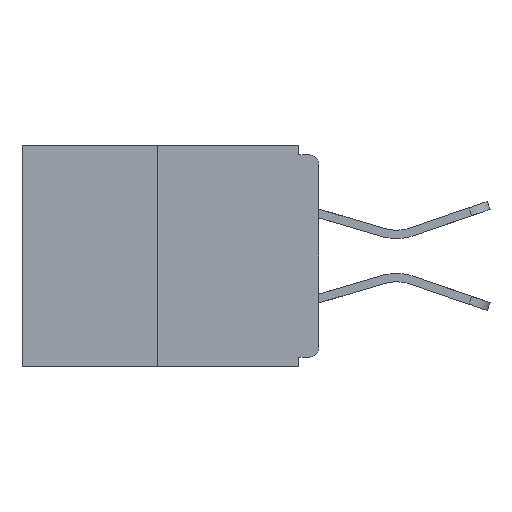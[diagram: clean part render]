
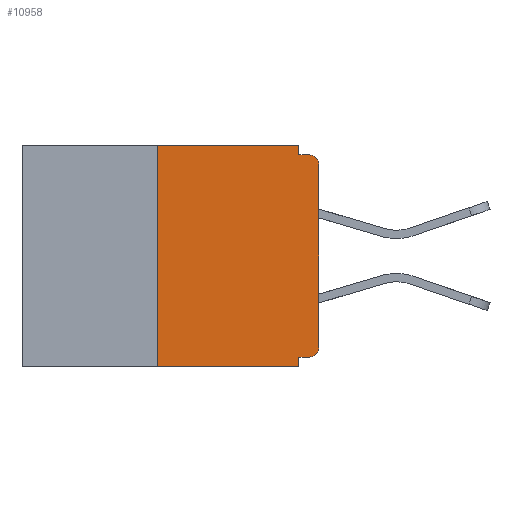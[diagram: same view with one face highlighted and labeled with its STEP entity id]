
A CAD part, left-side view. The second image highlights one B-rep face of the part: STEP entity #10958.
In plain terms, the highlighted planar face has unit normal (-1, 0, 0).
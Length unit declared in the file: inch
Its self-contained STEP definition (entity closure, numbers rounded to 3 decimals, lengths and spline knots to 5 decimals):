
#30 = VERTEX_POINT ( 'NONE', #23460 ) ;
#964 = AXIS2_PLACEMENT_3D ( 'NONE', #13225, #19103, #20833 ) ;
#1089 = VERTEX_POINT ( 'NONE', #25405 ) ;
#2059 = VECTOR ( 'NONE', #21796, 39.37008 ) ;
#2412 = VECTOR ( 'NONE', #14041, 39.37008 ) ;
#2723 = ORIENTED_EDGE ( 'NONE', *, *, #23331, .F. ) ;
#2793 = EDGE_CURVE ( 'NONE', #17201, #6545, #22233, .T. ) ;
#3294 = FACE_OUTER_BOUND ( 'NONE', #9768, .T. ) ;
#3352 = EDGE_CURVE ( 'NONE', #30, #1089, #16151, .T. ) ;
#3661 = CARTESIAN_POINT ( 'NONE',  ( 0., 0.015, -0.328 ) ) ;
#4598 = ORIENTED_EDGE ( 'NONE', *, *, #22551, .F. ) ;
#5006 = VECTOR ( 'NONE', #12530, 39.37008 ) ;
#5181 = DIRECTION ( 'NONE',  ( 0., 1., 0. ) ) ;
#5826 = VECTOR ( 'NONE', #22575, 39.37008 ) ;
#6290 = LINE ( 'NONE', #10565, #2412 ) ;
#6545 = VERTEX_POINT ( 'NONE', #8564 ) ;
#6872 = EDGE_CURVE ( 'NONE', #12479, #18015, #6290, .T. ) ;
#7161 = EDGE_CURVE ( 'NONE', #14339, #30, #17346, .T. ) ;
#7478 = DIRECTION ( 'NONE',  ( 0., 0., -1. ) ) ;
#7545 = PLANE ( 'NONE',  #19122 ) ;
#7570 = VERTEX_POINT ( 'NONE', #12518 ) ;
#7670 = CARTESIAN_POINT ( 'NONE',  ( 0., 0.46, 0. ) ) ;
#7829 = LINE ( 'NONE', #21703, #19369 ) ;
#7931 = DIRECTION ( 'NONE',  ( 0., 0., -1. ) ) ;
#8564 = CARTESIAN_POINT ( 'NONE',  ( 0., 0.015, -0.015 ) ) ;
#9344 = CARTESIAN_POINT ( 'NONE',  ( 0., 0.25, -0.343 ) ) ;
#9361 = ORIENTED_EDGE ( 'NONE', *, *, #24961, .T. ) ;
#9396 = ORIENTED_EDGE ( 'NONE', *, *, #2793, .T. ) ;
#9607 = CIRCLE ( 'NONE', #21958, 0.015 ) ;
#9642 = ORIENTED_EDGE ( 'NONE', *, *, #11290, .F. ) ;
#9716 = DIRECTION ( 'NONE',  ( 0., 0., 1. ) ) ;
#9768 = EDGE_LOOP ( 'NONE', ( #4598, #9642, #13772, #24468, #18959, #16604, #9361, #9396, #2723, #16376 ) ) ;
#9781 = VECTOR ( 'NONE', #24230, 39.37008 ) ;
#10565 = CARTESIAN_POINT ( 'NONE',  ( 0., 0.031, 0. ) ) ;
#10653 = CARTESIAN_POINT ( 'NONE',  ( 0., 0., -0.015 ) ) ;
#10958 = ADVANCED_FACE ( 'NONE', ( #3294 ), #7545, .F. ) ;
#11192 = DIRECTION ( 'NONE',  ( 0., 0., -1. ) ) ;
#11290 = EDGE_CURVE ( 'NONE', #21255, #24212, #7829, .T. ) ;
#11417 = LINE ( 'NONE', #21669, #2059 ) ;
#11774 = CARTESIAN_POINT ( 'NONE',  ( 0., 0., -0.03 ) ) ;
#12479 = VERTEX_POINT ( 'NONE', #24342 ) ;
#12518 = CARTESIAN_POINT ( 'NONE',  ( 0., 0., -0.313 ) ) ;
#12530 = DIRECTION ( 'NONE',  ( 0., -1., 0. ) ) ;
#13225 = CARTESIAN_POINT ( 'NONE',  ( 0., 0.015, -0.03 ) ) ;
#13479 = CARTESIAN_POINT ( 'NONE',  ( 0., 0.015, -0.313 ) ) ;
#13772 = ORIENTED_EDGE ( 'NONE', *, *, #23390, .T. ) ;
#13831 = DIRECTION ( 'NONE',  ( 1., 0., 0. ) ) ;
#13935 = VECTOR ( 'NONE', #5181, 39.37008 ) ;
#14041 = DIRECTION ( 'NONE',  ( 0., 0., -1. ) ) ;
#14100 = CARTESIAN_POINT ( 'NONE',  ( 0., 0., 0. ) ) ;
#14339 = VERTEX_POINT ( 'NONE', #3661 ) ;
#14469 = CARTESIAN_POINT ( 'NONE',  ( 0., 0.46, 0. ) ) ;
#15831 = CARTESIAN_POINT ( 'NONE',  ( 0., 0.031, -0.015 ) ) ;
#16151 = LINE ( 'NONE', #24278, #16752 ) ;
#16205 = EDGE_CURVE ( 'NONE', #14339, #7570, #9607, .T. ) ;
#16376 = ORIENTED_EDGE ( 'NONE', *, *, #6872, .F. ) ;
#16604 = ORIENTED_EDGE ( 'NONE', *, *, #16205, .T. ) ;
#16752 = VECTOR ( 'NONE', #7478, 39.37008 ) ;
#17201 = VERTEX_POINT ( 'NONE', #11774 ) ;
#17346 = LINE ( 'NONE', #23458, #13935 ) ;
#18015 = VERTEX_POINT ( 'NONE', #15831 ) ;
#18277 = LINE ( 'NONE', #10653, #5006 ) ;
#18959 = ORIENTED_EDGE ( 'NONE', *, *, #7161, .F. ) ;
#19103 = DIRECTION ( 'NONE',  ( -1., 0., 0. ) ) ;
#19122 = AXIS2_PLACEMENT_3D ( 'NONE', #7670, #13831, #7931 ) ;
#19369 = VECTOR ( 'NONE', #9716, 39.37008 ) ;
#20234 = LINE ( 'NONE', #14100, #9781 ) ;
#20833 = DIRECTION ( 'NONE',  ( 0., 0., -1. ) ) ;
#21060 = DIRECTION ( 'NONE',  ( -1., 0., 0. ) ) ;
#21255 = VERTEX_POINT ( 'NONE', #9344 ) ;
#21669 = CARTESIAN_POINT ( 'NONE',  ( 0., 0.46, -0.343 ) ) ;
#21703 = CARTESIAN_POINT ( 'NONE',  ( 0., 0.25, 0. ) ) ;
#21796 = DIRECTION ( 'NONE',  ( 0., -1., 0. ) ) ;
#21958 = AXIS2_PLACEMENT_3D ( 'NONE', #13479, #21060, #11192 ) ;
#22233 = CIRCLE ( 'NONE', #964, 0.015 ) ;
#22551 = EDGE_CURVE ( 'NONE', #24212, #12479, #24598, .T. ) ;
#22575 = DIRECTION ( 'NONE',  ( 0., -1., 0. ) ) ;
#23331 = EDGE_CURVE ( 'NONE', #18015, #6545, #18277, .T. ) ;
#23390 = EDGE_CURVE ( 'NONE', #21255, #1089, #11417, .T. ) ;
#23458 = CARTESIAN_POINT ( 'NONE',  ( 0., 0., -0.328 ) ) ;
#23460 = CARTESIAN_POINT ( 'NONE',  ( 0., 0.031, -0.328 ) ) ;
#24212 = VERTEX_POINT ( 'NONE', #24291 ) ;
#24230 = DIRECTION ( 'NONE',  ( 0., 0., 1. ) ) ;
#24278 = CARTESIAN_POINT ( 'NONE',  ( 0., 0.031, -0.343 ) ) ;
#24291 = CARTESIAN_POINT ( 'NONE',  ( 0., 0.25, 0. ) ) ;
#24342 = CARTESIAN_POINT ( 'NONE',  ( 0., 0.031, 0. ) ) ;
#24468 = ORIENTED_EDGE ( 'NONE', *, *, #3352, .F. ) ;
#24598 = LINE ( 'NONE', #14469, #5826 ) ;
#24961 = EDGE_CURVE ( 'NONE', #7570, #17201, #20234, .T. ) ;
#25405 = CARTESIAN_POINT ( 'NONE',  ( 0., 0.031, -0.343 ) ) ;
